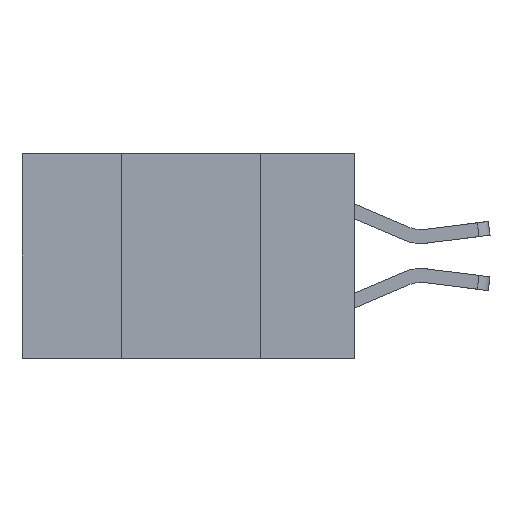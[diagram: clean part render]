
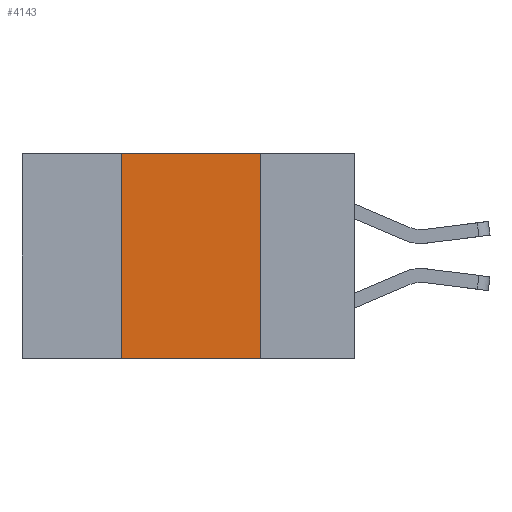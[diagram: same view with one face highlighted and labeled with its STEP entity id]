
A CAD part, left-side view. The second image highlights one B-rep face of the part: STEP entity #4143.
In plain terms, the highlighted planar face has unit normal (-1, 0, 0).
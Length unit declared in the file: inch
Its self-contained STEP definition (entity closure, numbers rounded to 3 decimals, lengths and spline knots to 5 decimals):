
#189 = AXIS2_PLACEMENT_3D ( 'NONE', #2941, #8073, #4821 ) ;
#452 = EDGE_CURVE ( 'NONE', #5499, #2929, #7519, .T. ) ;
#1229 = LINE ( 'NONE', #8963, #6021 ) ;
#1624 = CARTESIAN_POINT ( 'NONE',  ( 0., 0.42, 0. ) ) ;
#1696 = ORIENTED_EDGE ( 'NONE', *, *, #10745, .F. ) ;
#2075 = VERTEX_POINT ( 'NONE', #8492 ) ;
#2150 = EDGE_LOOP ( 'NONE', ( #6544, #12222, #1696, #7393 ) ) ;
#2929 = VERTEX_POINT ( 'NONE', #7924 ) ;
#2941 = CARTESIAN_POINT ( 'NONE',  ( 0., 0.6, 0. ) ) ;
#3314 = CARTESIAN_POINT ( 'NONE',  ( 0., 0.6, 0. ) ) ;
#3570 = DIRECTION ( 'NONE',  ( 0., 0., 1. ) ) ;
#3669 = CARTESIAN_POINT ( 'NONE',  ( 0., 0.17, 0. ) ) ;
#3965 = VECTOR ( 'NONE', #3570, 39.37008 ) ;
#4066 = VERTEX_POINT ( 'NONE', #6939 ) ;
#4143 = ADVANCED_FACE ( 'NONE', ( #4453 ), #6837, .F. ) ;
#4453 = FACE_OUTER_BOUND ( 'NONE', #2150, .T. ) ;
#4660 = DIRECTION ( 'NONE',  ( 0., -1., 0. ) ) ;
#4821 = DIRECTION ( 'NONE',  ( 0., 0., -1. ) ) ;
#4888 = EDGE_CURVE ( 'NONE', #2929, #2075, #6197, .T. ) ;
#5004 = VECTOR ( 'NONE', #4660, 39.37008 ) ;
#5499 = VERTEX_POINT ( 'NONE', #9348 ) ;
#6021 = VECTOR ( 'NONE', #9894, 39.37008 ) ;
#6197 = LINE ( 'NONE', #3669, #10879 ) ;
#6476 = LINE ( 'NONE', #1624, #3965 ) ;
#6544 = ORIENTED_EDGE ( 'NONE', *, *, #4888, .F. ) ;
#6837 = PLANE ( 'NONE',  #189 ) ;
#6939 = CARTESIAN_POINT ( 'NONE',  ( 0., 0.42, -0.37 ) ) ;
#7393 = ORIENTED_EDGE ( 'NONE', *, *, #10559, .T. ) ;
#7519 = LINE ( 'NONE', #3314, #5004 ) ;
#7924 = CARTESIAN_POINT ( 'NONE',  ( 0., 0.17, 0. ) ) ;
#8073 = DIRECTION ( 'NONE',  ( 1., 0., 0. ) ) ;
#8492 = CARTESIAN_POINT ( 'NONE',  ( 0., 0.17, -0.37 ) ) ;
#8963 = CARTESIAN_POINT ( 'NONE',  ( 0., 0.6, -0.37 ) ) ;
#9348 = CARTESIAN_POINT ( 'NONE',  ( 0., 0.42, 0. ) ) ;
#9361 = DIRECTION ( 'NONE',  ( 0., 0., -1. ) ) ;
#9894 = DIRECTION ( 'NONE',  ( 0., -1., 0. ) ) ;
#10559 = EDGE_CURVE ( 'NONE', #4066, #2075, #1229, .T. ) ;
#10745 = EDGE_CURVE ( 'NONE', #4066, #5499, #6476, .T. ) ;
#10879 = VECTOR ( 'NONE', #9361, 39.37008 ) ;
#12222 = ORIENTED_EDGE ( 'NONE', *, *, #452, .F. ) ;
